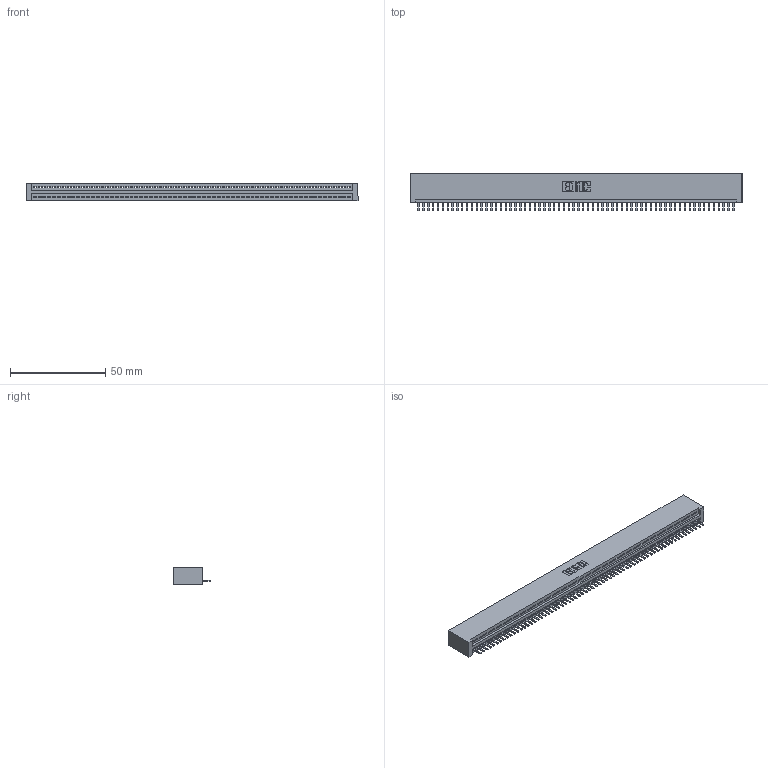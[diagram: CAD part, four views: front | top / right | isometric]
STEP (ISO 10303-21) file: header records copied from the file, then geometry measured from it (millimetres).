
FILE_DESCRIPTION (( 'STEP AP203' ), '1' );
FILE_NAME ('345-066-520-101.STEP', '2019-10-11T20:00:05', ( '' ), ( '' ), 'SwSTEP 2.0', 'SolidWorks 2016', '' );
FILE_SCHEMA (( 'CONFIG_CONTROL_DESIGN' ));
Length unit declared in the file: inch
Products named in the file (3): 345-292-001_345-293-120; 345-066-520-101; 345 Part_No Mounting Lugs
Assembly tree (67 placements, depth 2):
  345-066-520-101
    345 Part_No Mounting Lugs
    345-292-001_345-293-120  x66
Bounding box: 174.24 x 19.68 x 9.4 mm (x, y, z)
Volume: 17141 mm3; surface area: 22674 mm2
Topology: 67 solids, 67 shells, 4210 faces, 12461 edges, 8130 vertices
Faces by surface type: plane 2848, cylinder 1362
Entity records: 46279 total; most frequent: CARTESIAN_POINT 8034, ORIENTED_EDGE 8022, DIRECTION 6963, EDGE_CURVE 4011, VECTOR 3619, LINE 3619, VERTEX_POINT 2670, AXIS2_PLACEMENT_3D 1672
